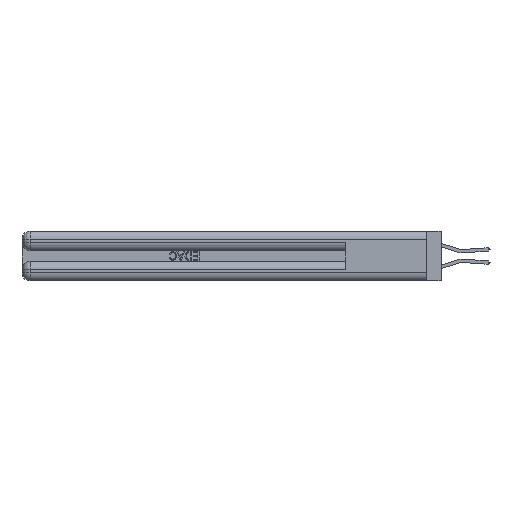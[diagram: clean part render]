
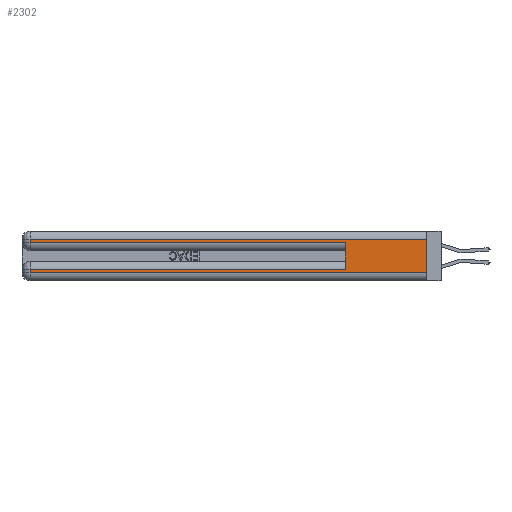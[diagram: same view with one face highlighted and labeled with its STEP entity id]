
A CAD part, left-side view. The second image highlights one B-rep face of the part: STEP entity #2302.
In plain terms, the highlighted planar face has unit normal (-1, 0, 0).
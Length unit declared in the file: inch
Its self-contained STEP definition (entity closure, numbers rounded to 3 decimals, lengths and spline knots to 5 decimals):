
#192 = ORIENTED_EDGE ( 'NONE', *, *, #28165, .T. ) ;
#530 = LINE ( 'NONE', #36142, #18548 ) ;
#1034 = DIRECTION ( 'NONE',  ( 0., 0., -1. ) ) ;
#1322 = DIRECTION ( 'NONE',  ( 0., 0., -1. ) ) ;
#1810 = CARTESIAN_POINT ( 'NONE',  ( 0., 0., 0.31 ) ) ;
#2302 = ADVANCED_FACE ( 'NONE', ( #27675 ), #29561, .F. ) ;
#2357 = EDGE_LOOP ( 'NONE', ( #9278, #41431, #192, #43116, #2968, #11532, #2461, #14361 ) ) ;
#2461 = ORIENTED_EDGE ( 'NONE', *, *, #25596, .T. ) ;
#2968 = ORIENTED_EDGE ( 'NONE', *, *, #38479, .F. ) ;
#4118 = CARTESIAN_POINT ( 'NONE',  ( 0., 2.94, 0.37 ) ) ;
#4226 = CARTESIAN_POINT ( 'NONE',  ( 0., 0.6, 0.285 ) ) ;
#5642 = CARTESIAN_POINT ( 'NONE',  ( 0., 2.94, 0.085 ) ) ;
#5941 = DIRECTION ( 'NONE',  ( 0., -1., 0. ) ) ;
#6034 = CARTESIAN_POINT ( 'NONE',  ( 0., 0., 0.31 ) ) ;
#6395 = VECTOR ( 'NONE', #12061, 39.37008 ) ;
#7053 = LINE ( 'NONE', #16307, #24954 ) ;
#7393 = VERTEX_POINT ( 'NONE', #18945 ) ;
#8431 = CARTESIAN_POINT ( 'NONE',  ( 0., 0.6, 0.145 ) ) ;
#8468 = CARTESIAN_POINT ( 'NONE',  ( 0., 0., 0.085 ) ) ;
#9063 = LINE ( 'NONE', #4118, #35213 ) ;
#9278 = ORIENTED_EDGE ( 'NONE', *, *, #37890, .F. ) ;
#10926 = VERTEX_POINT ( 'NONE', #30443 ) ;
#11308 = DIRECTION ( 'NONE',  ( 0., -1., 0. ) ) ;
#11532 = ORIENTED_EDGE ( 'NONE', *, *, #41413, .T. ) ;
#12061 = DIRECTION ( 'NONE',  ( 0., 0., 1. ) ) ;
#14361 = ORIENTED_EDGE ( 'NONE', *, *, #19307, .T. ) ;
#14707 = VERTEX_POINT ( 'NONE', #4226 ) ;
#16121 = AXIS2_PLACEMENT_3D ( 'NONE', #40053, #22566, #1034 ) ;
#16307 = CARTESIAN_POINT ( 'NONE',  ( 0., 2.94, 0.37 ) ) ;
#18032 = LINE ( 'NONE', #8468, #26396 ) ;
#18548 = VECTOR ( 'NONE', #11308, 39.37008 ) ;
#18945 = CARTESIAN_POINT ( 'NONE',  ( 0., 0., 0.06 ) ) ;
#19250 = CARTESIAN_POINT ( 'NONE',  ( 0., 0., 0.37 ) ) ;
#19307 = EDGE_CURVE ( 'NONE', #37738, #7393, #530, .T. ) ;
#20226 = VERTEX_POINT ( 'NONE', #1810 ) ;
#22566 = DIRECTION ( 'NONE',  ( 1., 0., 0. ) ) ;
#22645 = LINE ( 'NONE', #6034, #30977 ) ;
#22713 = LINE ( 'NONE', #19250, #31047 ) ;
#23797 = CARTESIAN_POINT ( 'NONE',  ( 0., 0., 0.285 ) ) ;
#24954 = VECTOR ( 'NONE', #37574, 39.37008 ) ;
#25105 = EDGE_CURVE ( 'NONE', #10926, #14707, #36649, .T. ) ;
#25596 = EDGE_CURVE ( 'NONE', #39310, #37738, #7053, .T. ) ;
#25734 = DIRECTION ( 'NONE',  ( 0., 0., -1. ) ) ;
#26396 = VECTOR ( 'NONE', #36933, 39.37008 ) ;
#26551 = LINE ( 'NONE', #8431, #6395 ) ;
#27675 = FACE_OUTER_BOUND ( 'NONE', #2357, .T. ) ;
#28165 = EDGE_CURVE ( 'NONE', #38898, #10926, #9063, .T. ) ;
#28337 = VECTOR ( 'NONE', #5941, 39.37008 ) ;
#29561 = PLANE ( 'NONE',  #16121 ) ;
#30443 = CARTESIAN_POINT ( 'NONE',  ( 0., 2.94, 0.285 ) ) ;
#30977 = VECTOR ( 'NONE', #34596, 39.37008 ) ;
#31047 = VECTOR ( 'NONE', #1322, 39.37008 ) ;
#34596 = DIRECTION ( 'NONE',  ( 0., 1., 0. ) ) ;
#35213 = VECTOR ( 'NONE', #25734, 39.37008 ) ;
#35601 = CARTESIAN_POINT ( 'NONE',  ( 0., 2.94, 0.06 ) ) ;
#36142 = CARTESIAN_POINT ( 'NONE',  ( 0., 0., 0.06 ) ) ;
#36649 = LINE ( 'NONE', #23797, #28337 ) ;
#36933 = DIRECTION ( 'NONE',  ( 0., 1., 0. ) ) ;
#37574 = DIRECTION ( 'NONE',  ( 0., 0., -1. ) ) ;
#37738 = VERTEX_POINT ( 'NONE', #35601 ) ;
#37890 = EDGE_CURVE ( 'NONE', #20226, #7393, #22713, .T. ) ;
#38479 = EDGE_CURVE ( 'NONE', #41691, #14707, #26551, .T. ) ;
#38898 = VERTEX_POINT ( 'NONE', #39171 ) ;
#39171 = CARTESIAN_POINT ( 'NONE',  ( 0., 2.94, 0.31 ) ) ;
#39310 = VERTEX_POINT ( 'NONE', #5642 ) ;
#39888 = EDGE_CURVE ( 'NONE', #20226, #38898, #22645, .T. ) ;
#40053 = CARTESIAN_POINT ( 'NONE',  ( 0., 0., 0.37 ) ) ;
#41413 = EDGE_CURVE ( 'NONE', #41691, #39310, #18032, .T. ) ;
#41431 = ORIENTED_EDGE ( 'NONE', *, *, #39888, .T. ) ;
#41691 = VERTEX_POINT ( 'NONE', #42109 ) ;
#42109 = CARTESIAN_POINT ( 'NONE',  ( 0., 0.6, 0.085 ) ) ;
#43116 = ORIENTED_EDGE ( 'NONE', *, *, #25105, .T. ) ;
